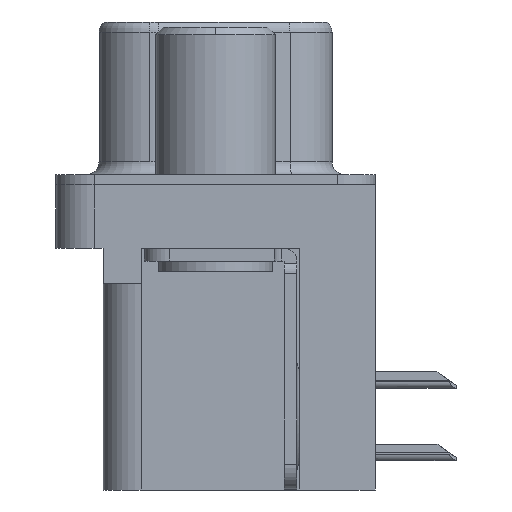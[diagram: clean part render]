
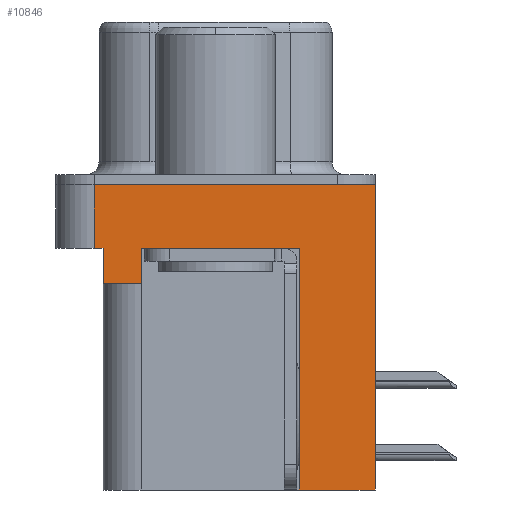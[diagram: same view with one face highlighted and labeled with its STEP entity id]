
A CAD part, left-side view. The second image highlights one B-rep face of the part: STEP entity #10846.
In plain terms, the highlighted planar face has unit normal (-1, 0, 0).
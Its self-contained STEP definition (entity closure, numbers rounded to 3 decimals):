
#4 = DIRECTION ( 'NONE',  ( 0., 1., 0. ) ) ;
#52 = LINE ( 'NONE', #12014, #8412 ) ;
#536 = DIRECTION ( 'NONE',  ( 0., -1., 0. ) ) ;
#670 = CARTESIAN_POINT ( 'NONE',  ( -3., 2.895, -3.9 ) ) ;
#1247 = LINE ( 'NONE', #11851, #11104 ) ;
#1846 = VECTOR ( 'NONE', #4, 1000. ) ;
#1864 = CARTESIAN_POINT ( 'NONE',  ( -3., 2.895, -2.5 ) ) ;
#1916 = CARTESIAN_POINT ( 'NONE',  ( -3., -3.295, -12. ) ) ;
#2197 = EDGE_CURVE ( 'NONE', #19973, #17462, #16108, .T. ) ;
#2301 = EDGE_CURVE ( 'NONE', #23879, #12381, #1247, .T. ) ;
#2566 = CARTESIAN_POINT ( 'NONE',  ( -3., 4.775, 0. ) ) ;
#2897 = CARTESIAN_POINT ( 'NONE',  ( -3., -6.275, -2.5 ) ) ;
#3535 = CARTESIAN_POINT ( 'NONE',  ( -3., -6.275, 0. ) ) ;
#3704 = VECTOR ( 'NONE', #19521, 1000. ) ;
#3894 = DIRECTION ( 'NONE',  ( -1., 0., 0. ) ) ;
#3980 = EDGE_CURVE ( 'NONE', #19973, #6786, #23766, .T. ) ;
#4131 = CARTESIAN_POINT ( 'NONE',  ( -3., -3.295, -12. ) ) ;
#4806 = DIRECTION ( 'NONE',  ( 0., 0., 1. ) ) ;
#5514 = EDGE_CURVE ( 'NONE', #15686, #6786, #18607, .T. ) ;
#5755 = ORIENTED_EDGE ( 'NONE', *, *, #24590, .F. ) ;
#6775 = ORIENTED_EDGE ( 'NONE', *, *, #2197, .F. ) ;
#6786 = VERTEX_POINT ( 'NONE', #3535 ) ;
#6940 = EDGE_CURVE ( 'NONE', #18046, #11136, #21519, .T. ) ;
#7711 = CARTESIAN_POINT ( 'NONE',  ( -3., 4.425, -3.9 ) ) ;
#8100 = DIRECTION ( 'NONE',  ( 0., -1., 0. ) ) ;
#8412 = VECTOR ( 'NONE', #11774, 1000. ) ;
#9587 = LINE ( 'NONE', #4131, #11080 ) ;
#9636 = ORIENTED_EDGE ( 'NONE', *, *, #15136, .T. ) ;
#9814 = DIRECTION ( 'NONE',  ( 0., 1., 0. ) ) ;
#9917 = ORIENTED_EDGE ( 'NONE', *, *, #16676, .F. ) ;
#10383 = CARTESIAN_POINT ( 'NONE',  ( -3., 4.425, -2.5 ) ) ;
#10796 = LINE ( 'NONE', #11560, #18171 ) ;
#10846 = ADVANCED_FACE ( 'NONE', ( #13169 ), #20727, .T. ) ;
#11080 = VECTOR ( 'NONE', #11933, 1000. ) ;
#11104 = VECTOR ( 'NONE', #8100, 1000. ) ;
#11112 = AXIS2_PLACEMENT_3D ( 'NONE', #11537, #3894, #11613 ) ;
#11136 = VERTEX_POINT ( 'NONE', #10383 ) ;
#11537 = CARTESIAN_POINT ( 'NONE',  ( -3., -6.275, -2.5 ) ) ;
#11560 = CARTESIAN_POINT ( 'NONE',  ( -3., 4.425, -3.9 ) ) ;
#11613 = DIRECTION ( 'NONE',  ( 0., 0., 1. ) ) ;
#11640 = CARTESIAN_POINT ( 'NONE',  ( -3., -6.275, 0. ) ) ;
#11737 = LINE ( 'NONE', #13925, #3704 ) ;
#11774 = DIRECTION ( 'NONE',  ( 0., 0., 1. ) ) ;
#11851 = CARTESIAN_POINT ( 'NONE',  ( -3., -6.275, -2.5 ) ) ;
#11933 = DIRECTION ( 'NONE',  ( 0., 0., 1. ) ) ;
#12014 = CARTESIAN_POINT ( 'NONE',  ( -3., 4.775, -2.5 ) ) ;
#12253 = CARTESIAN_POINT ( 'NONE',  ( -3., -3.295, -2.5 ) ) ;
#12381 = VERTEX_POINT ( 'NONE', #12253 ) ;
#12867 = ORIENTED_EDGE ( 'NONE', *, *, #3980, .T. ) ;
#13169 = FACE_OUTER_BOUND ( 'NONE', #21300, .T. ) ;
#13254 = CARTESIAN_POINT ( 'NONE',  ( -3., -3.295, -12. ) ) ;
#13912 = ORIENTED_EDGE ( 'NONE', *, *, #6940, .F. ) ;
#13925 = CARTESIAN_POINT ( 'NONE',  ( -3., -6.275, -2.5 ) ) ;
#13984 = VECTOR ( 'NONE', #19612, 1000. ) ;
#14009 = ORIENTED_EDGE ( 'NONE', *, *, #18339, .T. ) ;
#14100 = ORIENTED_EDGE ( 'NONE', *, *, #5514, .F. ) ;
#14578 = LINE ( 'NONE', #670, #13984 ) ;
#14905 = VECTOR ( 'NONE', #4806, 1000. ) ;
#15136 = EDGE_CURVE ( 'NONE', #23538, #11136, #11737, .T. ) ;
#15686 = VERTEX_POINT ( 'NONE', #2566 ) ;
#16108 = LINE ( 'NONE', #1916, #1846 ) ;
#16676 = EDGE_CURVE ( 'NONE', #20738, #18046, #10796, .T. ) ;
#16929 = CARTESIAN_POINT ( 'NONE',  ( -3., -6.275, -12. ) ) ;
#17462 = VERTEX_POINT ( 'NONE', #13254 ) ;
#18046 = VERTEX_POINT ( 'NONE', #7711 ) ;
#18115 = ORIENTED_EDGE ( 'NONE', *, *, #20521, .F. ) ;
#18171 = VECTOR ( 'NONE', #9814, 1000. ) ;
#18339 = EDGE_CURVE ( 'NONE', #20738, #23879, #14578, .T. ) ;
#18403 = ORIENTED_EDGE ( 'NONE', *, *, #2301, .T. ) ;
#18607 = LINE ( 'NONE', #11640, #20980 ) ;
#19521 = DIRECTION ( 'NONE',  ( 0., -1., 0. ) ) ;
#19612 = DIRECTION ( 'NONE',  ( 0., 0., 1. ) ) ;
#19654 = CARTESIAN_POINT ( 'NONE',  ( -3., 4.775, -2.5 ) ) ;
#19973 = VERTEX_POINT ( 'NONE', #16929 ) ;
#20521 = EDGE_CURVE ( 'NONE', #23538, #15686, #52, .T. ) ;
#20727 = PLANE ( 'NONE',  #11112 ) ;
#20738 = VERTEX_POINT ( 'NONE', #21599 ) ;
#20980 = VECTOR ( 'NONE', #536, 1000. ) ;
#21268 = CARTESIAN_POINT ( 'NONE',  ( -3., 4.425, -3.9 ) ) ;
#21300 = EDGE_LOOP ( 'NONE', ( #14100, #18115, #9636, #13912, #9917, #14009, #18403, #5755, #6775, #12867 ) ) ;
#21519 = LINE ( 'NONE', #21268, #22967 ) ;
#21599 = CARTESIAN_POINT ( 'NONE',  ( -3., 2.895, -3.9 ) ) ;
#22967 = VECTOR ( 'NONE', #23130, 1000. ) ;
#23130 = DIRECTION ( 'NONE',  ( 0., 0., 1. ) ) ;
#23538 = VERTEX_POINT ( 'NONE', #19654 ) ;
#23766 = LINE ( 'NONE', #2897, #14905 ) ;
#23879 = VERTEX_POINT ( 'NONE', #1864 ) ;
#24590 = EDGE_CURVE ( 'NONE', #17462, #12381, #9587, .T. ) ;
